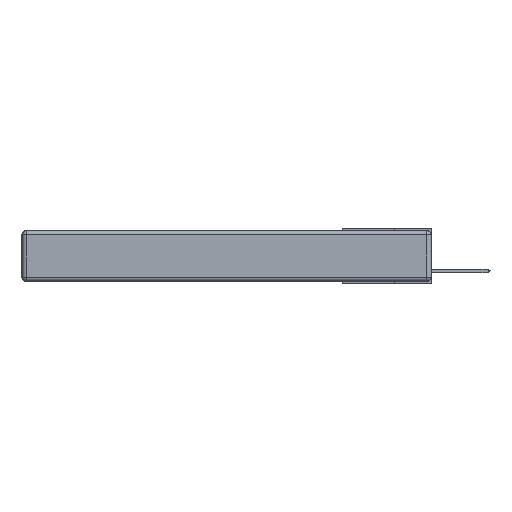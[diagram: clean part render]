
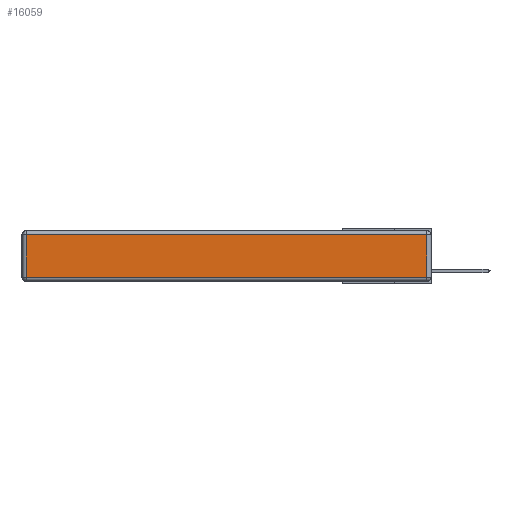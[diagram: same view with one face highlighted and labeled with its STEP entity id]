
A CAD part, left-side view. The second image highlights one B-rep face of the part: STEP entity #16059.
In plain terms, the highlighted planar face has unit normal (-1, 0, 0).
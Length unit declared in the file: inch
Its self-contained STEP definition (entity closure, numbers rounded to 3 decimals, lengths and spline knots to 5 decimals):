
#114 = VERTEX_POINT ( 'NONE', #12319 ) ;
#503 = CARTESIAN_POINT ( 'NONE',  ( 0., 2.75, -0.03 ) ) ;
#1095 = CARTESIAN_POINT ( 'NONE',  ( 0., 0.03, -0.343 ) ) ;
#1186 = CARTESIAN_POINT ( 'NONE',  ( 0., 2.72, -0.343 ) ) ;
#2018 = ORIENTED_EDGE ( 'NONE', *, *, #27464, .T. ) ;
#3877 = CARTESIAN_POINT ( 'NONE',  ( 0., 0., -0.313 ) ) ;
#4333 = ORIENTED_EDGE ( 'NONE', *, *, #32435, .T. ) ;
#6071 = LINE ( 'NONE', #1186, #30335 ) ;
#9674 = VECTOR ( 'NONE', #29205, 39.37008 ) ;
#9875 = VECTOR ( 'NONE', #19429, 39.37008 ) ;
#10422 = CARTESIAN_POINT ( 'NONE',  ( 0., 2.72, -0.313 ) ) ;
#10712 = VERTEX_POINT ( 'NONE', #11070 ) ;
#11070 = CARTESIAN_POINT ( 'NONE',  ( 0., 2.72, -0.03 ) ) ;
#11855 = CARTESIAN_POINT ( 'NONE',  ( 0., 0., -0.343 ) ) ;
#12268 = VERTEX_POINT ( 'NONE', #10422 ) ;
#12319 = CARTESIAN_POINT ( 'NONE',  ( 0., 0.03, -0.03 ) ) ;
#13085 = FACE_OUTER_BOUND ( 'NONE', #31339, .T. ) ;
#15461 = VERTEX_POINT ( 'NONE', #33593 ) ;
#16059 = ADVANCED_FACE ( 'NONE', ( #13085 ), #33170, .T. ) ;
#16831 = AXIS2_PLACEMENT_3D ( 'NONE', #11855, #20066, #33284 ) ;
#18505 = LINE ( 'NONE', #1095, #9875 ) ;
#19429 = DIRECTION ( 'NONE',  ( 0., 0., 1. ) ) ;
#20066 = DIRECTION ( 'NONE',  ( -1., 0., 0. ) ) ;
#25071 = EDGE_CURVE ( 'NONE', #114, #10712, #30632, .T. ) ;
#27464 = EDGE_CURVE ( 'NONE', #15461, #114, #18505, .T. ) ;
#29205 = DIRECTION ( 'NONE',  ( 0., 1., 0. ) ) ;
#30107 = EDGE_CURVE ( 'NONE', #12268, #15461, #30947, .T. ) ;
#30335 = VECTOR ( 'NONE', #32164, 39.37008 ) ;
#30632 = LINE ( 'NONE', #503, #9674 ) ;
#30947 = LINE ( 'NONE', #3877, #32187 ) ;
#30962 = ORIENTED_EDGE ( 'NONE', *, *, #25071, .T. ) ;
#31339 = EDGE_LOOP ( 'NONE', ( #33344, #2018, #30962, #4333 ) ) ;
#32164 = DIRECTION ( 'NONE',  ( 0., 0., -1. ) ) ;
#32187 = VECTOR ( 'NONE', #32500, 39.37008 ) ;
#32435 = EDGE_CURVE ( 'NONE', #10712, #12268, #6071, .T. ) ;
#32500 = DIRECTION ( 'NONE',  ( 0., -1., 0. ) ) ;
#33170 = PLANE ( 'NONE',  #16831 ) ;
#33284 = DIRECTION ( 'NONE',  ( 0., 0., 1. ) ) ;
#33344 = ORIENTED_EDGE ( 'NONE', *, *, #30107, .T. ) ;
#33593 = CARTESIAN_POINT ( 'NONE',  ( 0., 0.03, -0.313 ) ) ;
